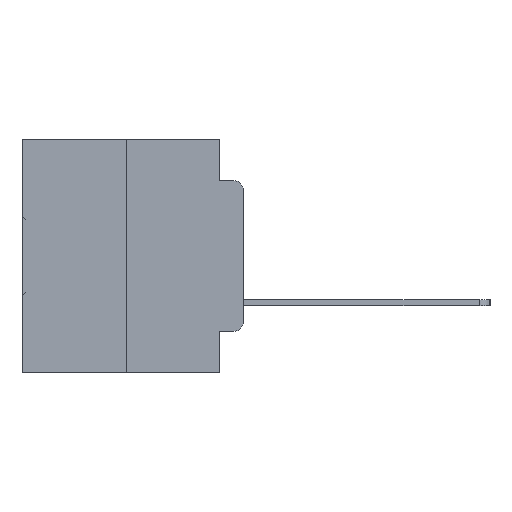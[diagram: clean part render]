
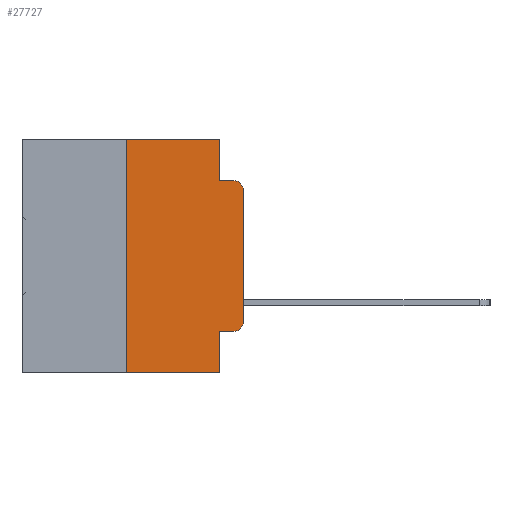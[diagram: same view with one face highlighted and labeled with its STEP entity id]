
A CAD part, left-side view. The second image highlights one B-rep face of the part: STEP entity #27727.
In plain terms, the highlighted planar face has unit normal (-1, 0, 0).
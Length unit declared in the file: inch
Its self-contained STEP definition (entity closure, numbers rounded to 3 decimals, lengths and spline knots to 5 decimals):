
#414 = EDGE_LOOP ( 'NONE', ( #29867, #3452, #17636, #19302, #26249, #15581, #22551, #10995, #18068, #25049 ) ) ;
#526 = LINE ( 'NONE', #27036, #20198 ) ;
#1142 = DIRECTION ( 'NONE',  ( 0., 0., -1. ) ) ;
#2117 = LINE ( 'NONE', #14579, #13911 ) ;
#2402 = CARTESIAN_POINT ( 'NONE',  ( 0., 0.02, -0.4115 ) ) ;
#3313 = CARTESIAN_POINT ( 'NONE',  ( 0., 0., -0.3915 ) ) ;
#3452 = ORIENTED_EDGE ( 'NONE', *, *, #26294, .T. ) ;
#4870 = CARTESIAN_POINT ( 'NONE',  ( 0., 0.02, -0.1085 ) ) ;
#5517 = CIRCLE ( 'NONE', #17446, 0.02 ) ;
#5537 = CARTESIAN_POINT ( 'NONE',  ( 0., 0.051, 0. ) ) ;
#5870 = VECTOR ( 'NONE', #18791, 39.37008 ) ;
#6814 = LINE ( 'NONE', #15864, #13886 ) ;
#7487 = CARTESIAN_POINT ( 'NONE',  ( 0., 0., 0. ) ) ;
#7598 = DIRECTION ( 'NONE',  ( 0., 0., -1. ) ) ;
#8046 = CARTESIAN_POINT ( 'NONE',  ( 0., 0.051, -0.5 ) ) ;
#8629 = DIRECTION ( 'NONE',  ( 0., -1., 0. ) ) ;
#8687 = VERTEX_POINT ( 'NONE', #9819 ) ;
#8788 = CARTESIAN_POINT ( 'NONE',  ( 0., 0.051, 0. ) ) ;
#9230 = LINE ( 'NONE', #21866, #21575 ) ;
#9819 = CARTESIAN_POINT ( 'NONE',  ( 0., 0.25, 0. ) ) ;
#10112 = VERTEX_POINT ( 'NONE', #19270 ) ;
#10212 = VECTOR ( 'NONE', #29291, 39.37008 ) ;
#10506 = DIRECTION ( 'NONE',  ( 0., -1., 0. ) ) ;
#10995 = ORIENTED_EDGE ( 'NONE', *, *, #19290, .F. ) ;
#11022 = LINE ( 'NONE', #26698, #10212 ) ;
#11083 = VERTEX_POINT ( 'NONE', #25942 ) ;
#11132 = DIRECTION ( 'NONE',  ( 0., -1., 0. ) ) ;
#11711 = LINE ( 'NONE', #7487, #12545 ) ;
#11840 = CARTESIAN_POINT ( 'NONE',  ( 0., 0.25, 0. ) ) ;
#12545 = VECTOR ( 'NONE', #25934, 39.37008 ) ;
#12822 = CARTESIAN_POINT ( 'NONE',  ( 0., 0.051, -0.4115 ) ) ;
#13886 = VECTOR ( 'NONE', #10506, 39.37008 ) ;
#13911 = VECTOR ( 'NONE', #1142, 39.37008 ) ;
#13924 = CARTESIAN_POINT ( 'NONE',  ( 0., 0.02, -0.3915 ) ) ;
#13983 = EDGE_CURVE ( 'NONE', #21829, #34195, #5517, .T. ) ;
#14147 = CARTESIAN_POINT ( 'NONE',  ( 0., 0.473, 0. ) ) ;
#14265 = DIRECTION ( 'NONE',  ( 0., 0., -1. ) ) ;
#14571 = DIRECTION ( 'NONE',  ( 0., 0., 1. ) ) ;
#14579 = CARTESIAN_POINT ( 'NONE',  ( 0., 0.051, 0. ) ) ;
#14628 = LINE ( 'NONE', #5537, #5870 ) ;
#15092 = AXIS2_PLACEMENT_3D ( 'NONE', #4870, #23392, #7598 ) ;
#15581 = ORIENTED_EDGE ( 'NONE', *, *, #20993, .F. ) ;
#15740 = EDGE_CURVE ( 'NONE', #25464, #21829, #526, .T. ) ;
#15864 = CARTESIAN_POINT ( 'NONE',  ( 0., 0.473, -0.5 ) ) ;
#16587 = DIRECTION ( 'NONE',  ( 0., 0., -1. ) ) ;
#17446 = AXIS2_PLACEMENT_3D ( 'NONE', #13924, #32134, #16587 ) ;
#17636 = ORIENTED_EDGE ( 'NONE', *, *, #24553, .F. ) ;
#17976 = EDGE_CURVE ( 'NONE', #10112, #23104, #6814, .T. ) ;
#18068 = ORIENTED_EDGE ( 'NONE', *, *, #15740, .T. ) ;
#18791 = DIRECTION ( 'NONE',  ( 0., 0., -1. ) ) ;
#18879 = AXIS2_PLACEMENT_3D ( 'NONE', #14147, #29899, #14265 ) ;
#19270 = CARTESIAN_POINT ( 'NONE',  ( 0., 0.25, -0.5 ) ) ;
#19290 = EDGE_CURVE ( 'NONE', #25464, #23104, #14628, .T. ) ;
#19302 = ORIENTED_EDGE ( 'NONE', *, *, #22779, .F. ) ;
#20198 = VECTOR ( 'NONE', #11132, 39.37008 ) ;
#20815 = FACE_OUTER_BOUND ( 'NONE', #414, .T. ) ;
#20993 = EDGE_CURVE ( 'NONE', #10112, #8687, #21443, .T. ) ;
#21443 = LINE ( 'NONE', #11840, #32795 ) ;
#21575 = VECTOR ( 'NONE', #8629, 39.37008 ) ;
#21829 = VERTEX_POINT ( 'NONE', #2402 ) ;
#21866 = CARTESIAN_POINT ( 'NONE',  ( 0., 0.051, -0.0885 ) ) ;
#22551 = ORIENTED_EDGE ( 'NONE', *, *, #17976, .T. ) ;
#22643 = VERTEX_POINT ( 'NONE', #8788 ) ;
#22779 = EDGE_CURVE ( 'NONE', #22643, #11083, #2117, .T. ) ;
#23104 = VERTEX_POINT ( 'NONE', #8046 ) ;
#23392 = DIRECTION ( 'NONE',  ( -1., 0., 0. ) ) ;
#24553 = EDGE_CURVE ( 'NONE', #11083, #33181, #9230, .T. ) ;
#24710 = PLANE ( 'NONE',  #18879 ) ;
#25032 = CARTESIAN_POINT ( 'NONE',  ( 0., 0., -0.1085 ) ) ;
#25049 = ORIENTED_EDGE ( 'NONE', *, *, #13983, .T. ) ;
#25464 = VERTEX_POINT ( 'NONE', #12822 ) ;
#25849 = VERTEX_POINT ( 'NONE', #25032 ) ;
#25934 = DIRECTION ( 'NONE',  ( 0., 0., 1. ) ) ;
#25942 = CARTESIAN_POINT ( 'NONE',  ( 0., 0.051, -0.0885 ) ) ;
#26249 = ORIENTED_EDGE ( 'NONE', *, *, #32328, .F. ) ;
#26294 = EDGE_CURVE ( 'NONE', #25849, #33181, #29666, .T. ) ;
#26698 = CARTESIAN_POINT ( 'NONE',  ( 0., 0.473, 0. ) ) ;
#27036 = CARTESIAN_POINT ( 'NONE',  ( 0., 0.051, -0.4115 ) ) ;
#27727 = ADVANCED_FACE ( 'NONE', ( #20815 ), #24710, .F. ) ;
#28004 = EDGE_CURVE ( 'NONE', #34195, #25849, #11711, .T. ) ;
#28101 = CARTESIAN_POINT ( 'NONE',  ( 0., 0.02, -0.0885 ) ) ;
#29291 = DIRECTION ( 'NONE',  ( 0., -1., 0. ) ) ;
#29666 = CIRCLE ( 'NONE', #15092, 0.02 ) ;
#29867 = ORIENTED_EDGE ( 'NONE', *, *, #28004, .T. ) ;
#29899 = DIRECTION ( 'NONE',  ( 1., 0., 0. ) ) ;
#32134 = DIRECTION ( 'NONE',  ( -1., 0., 0. ) ) ;
#32328 = EDGE_CURVE ( 'NONE', #8687, #22643, #11022, .T. ) ;
#32795 = VECTOR ( 'NONE', #14571, 39.37008 ) ;
#33181 = VERTEX_POINT ( 'NONE', #28101 ) ;
#34195 = VERTEX_POINT ( 'NONE', #3313 ) ;
